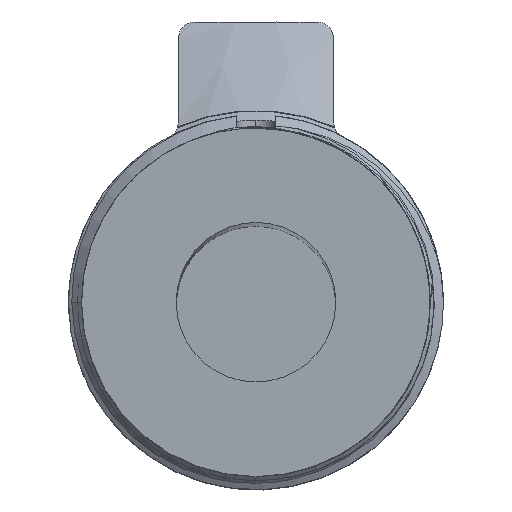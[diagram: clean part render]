
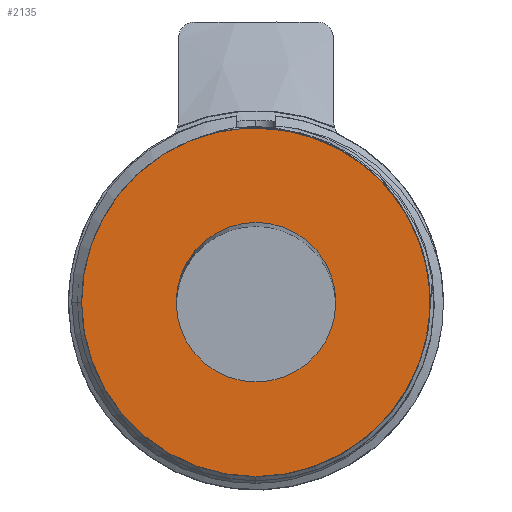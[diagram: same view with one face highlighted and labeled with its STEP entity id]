
A CAD part, top view. The second image highlights one B-rep face of the part: STEP entity #2135.
In plain terms, the highlighted planar face has unit normal (0, 0, 1).
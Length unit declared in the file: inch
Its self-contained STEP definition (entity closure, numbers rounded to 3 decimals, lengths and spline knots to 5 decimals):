
#702 = DIRECTION ( 'NONE',  ( -1., 0., 0. ) ) ;
#718 = DIRECTION ( 'NONE',  ( 0., 0., 1. ) ) ;
#754 = CARTESIAN_POINT ( 'NONE',  ( 0., 0., -0.61148 ) ) ;
#1189 = AXIS2_PLACEMENT_3D ( 'NONE', #754, #718, #702 ) ;
#1603 = EDGE_CURVE ( 'NONE', #5275, #23078, #8445, .T. ) ;
#1976 = AXIS2_PLACEMENT_3D ( 'NONE', #15244, #15223, #15192 ) ;
#2135 = ADVANCED_FACE ( 'NONE', ( #5750, #10252 ), #12650, .F. ) ;
#2254 = VERTEX_POINT ( 'NONE', #11111 ) ;
#2513 = AXIS2_PLACEMENT_3D ( 'NONE', #10642, #23355, #12513 ) ;
#2753 = DIRECTION ( 'NONE',  ( 1., 0., 0. ) ) ;
#2784 = DIRECTION ( 'NONE',  ( 0., 0., 1. ) ) ;
#2831 = CARTESIAN_POINT ( 'NONE',  ( 0., 0., -0.61148 ) ) ;
#2864 = CARTESIAN_POINT ( 'NONE',  ( -0.03437, 0.54536, -0.61148 ) ) ;
#3596 = EDGE_LOOP ( 'NONE', ( #18310, #4733 ) ) ;
#4570 = CIRCLE ( 'NONE', #1976, 0.25 ) ;
#4733 = ORIENTED_EDGE ( 'NONE', *, *, #6120, .F. ) ;
#5201 = EDGE_CURVE ( 'NONE', #23078, #9581, #8021, .T. ) ;
#5275 = VERTEX_POINT ( 'NONE', #20963 ) ;
#5374 = VERTEX_POINT ( 'NONE', #21486 ) ;
#5439 = EDGE_CURVE ( 'NONE', #9581, #2254, #22182, .T. ) ;
#5463 = ORIENTED_EDGE ( 'NONE', *, *, #1603, .T. ) ;
#5473 = AXIS2_PLACEMENT_3D ( 'NONE', #11631, #11604, #11600 ) ;
#5750 = FACE_OUTER_BOUND ( 'NONE', #21559, .T. ) ;
#6120 = EDGE_CURVE ( 'NONE', #18242, #16100, #4570, .T. ) ;
#7028 = ORIENTED_EDGE ( 'NONE', *, *, #21829, .T. ) ;
#7811 = CARTESIAN_POINT ( 'NONE',  ( 0., 0.54544, -0.61148 ) ) ;
#8021 = B_SPLINE_CURVE_WITH_KNOTS ( 'NONE', 3,
 ( #8293, #13998, #19482, #2864 ),
 .UNSPECIFIED., .F., .F.,
 ( 4, 4 ),
 ( 0.00007, 0.00094 ),
 .UNSPECIFIED. ) ;
#8293 = CARTESIAN_POINT ( 'NONE',  ( 0., 0.54544, -0.61148 ) ) ;
#8445 = B_SPLINE_CURVE_WITH_KNOTS ( 'NONE', 3,
 ( #21094, #21117, #21123, #21066 ),
 .UNSPECIFIED., .F., .F.,
 ( 4, 4 ),
 ( 0.01009, 0.01096 ),
 .UNSPECIFIED. ) ;
#9581 = VERTEX_POINT ( 'NONE', #18763 ) ;
#10252 = FACE_BOUND ( 'NONE', #3596, .T. ) ;
#10642 = CARTESIAN_POINT ( 'NONE',  ( 0., 0., -0.61148 ) ) ;
#10903 = EDGE_CURVE ( 'NONE', #16100, #18242, #22102, .T. ) ;
#11098 = DIRECTION ( 'NONE',  ( 0., 0., 1. ) ) ;
#11111 = CARTESIAN_POINT ( 'NONE',  ( -0.54644, 0., -0.61148 ) ) ;
#11600 = DIRECTION ( 'NONE',  ( -1., 0., 0. ) ) ;
#11604 = DIRECTION ( 'NONE',  ( 0., 0., -1. ) ) ;
#11631 = CARTESIAN_POINT ( 'NONE',  ( 0.55299, -0.5512, -0.61148 ) ) ;
#12104 = CIRCLE ( 'NONE', #2513, 0.54644 ) ;
#12513 = DIRECTION ( 'NONE',  ( -1., 0., 0. ) ) ;
#12650 = PLANE ( 'NONE',  #5473 ) ;
#13998 = CARTESIAN_POINT ( 'NONE',  ( -0.01146, 0.54576, -0.61148 ) ) ;
#14343 = ORIENTED_EDGE ( 'NONE', *, *, #5201, .T. ) ;
#15192 = DIRECTION ( 'NONE',  ( 1., 0., 0. ) ) ;
#15223 = DIRECTION ( 'NONE',  ( 0., 0., 1. ) ) ;
#15244 = CARTESIAN_POINT ( 'NONE',  ( 0., 0., -0.61148 ) ) ;
#16100 = VERTEX_POINT ( 'NONE', #16934 ) ;
#16690 = CARTESIAN_POINT ( 'NONE',  ( 0.25, 0., -0.61148 ) ) ;
#16934 = CARTESIAN_POINT ( 'NONE',  ( -0.25, 0., -0.61148 ) ) ;
#17939 = AXIS2_PLACEMENT_3D ( 'NONE', #2831, #2784, #2753 ) ;
#18242 = VERTEX_POINT ( 'NONE', #16690 ) ;
#18310 = ORIENTED_EDGE ( 'NONE', *, *, #10903, .F. ) ;
#18763 = CARTESIAN_POINT ( 'NONE',  ( -0.03437, 0.54536, -0.61148 ) ) ;
#19482 = CARTESIAN_POINT ( 'NONE',  ( -0.02292, 0.54574, -0.61148 ) ) ;
#19591 = EDGE_CURVE ( 'NONE', #2254, #5374, #22309, .T. ) ;
#20193 = AXIS2_PLACEMENT_3D ( 'NONE', #21966, #11098, #23767 ) ;
#20963 = CARTESIAN_POINT ( 'NONE',  ( 0.03437, 0.54536, -0.61148 ) ) ;
#21066 = CARTESIAN_POINT ( 'NONE',  ( 0., 0.54544, -0.61148 ) ) ;
#21094 = CARTESIAN_POINT ( 'NONE',  ( 0.03437, 0.54536, -0.61148 ) ) ;
#21117 = CARTESIAN_POINT ( 'NONE',  ( 0.02292, 0.54574, -0.61148 ) ) ;
#21123 = CARTESIAN_POINT ( 'NONE',  ( 0.01147, 0.54577, -0.61148 ) ) ;
#21486 = CARTESIAN_POINT ( 'NONE',  ( 0.54644, 0., -0.61148 ) ) ;
#21559 = EDGE_LOOP ( 'NONE', ( #14343, #21754, #21637, #7028, #5463 ) ) ;
#21637 = ORIENTED_EDGE ( 'NONE', *, *, #19591, .T. ) ;
#21754 = ORIENTED_EDGE ( 'NONE', *, *, #5439, .T. ) ;
#21829 = EDGE_CURVE ( 'NONE', #5374, #5275, #12104, .T. ) ;
#21966 = CARTESIAN_POINT ( 'NONE',  ( 0., 0., -0.61148 ) ) ;
#22102 = CIRCLE ( 'NONE', #17939, 0.25 ) ;
#22182 = CIRCLE ( 'NONE', #1189, 0.54644 ) ;
#22309 = CIRCLE ( 'NONE', #20193, 0.54644 ) ;
#23078 = VERTEX_POINT ( 'NONE', #7811 ) ;
#23355 = DIRECTION ( 'NONE',  ( 0., 0., 1. ) ) ;
#23767 = DIRECTION ( 'NONE',  ( -1., 0., 0. ) ) ;
